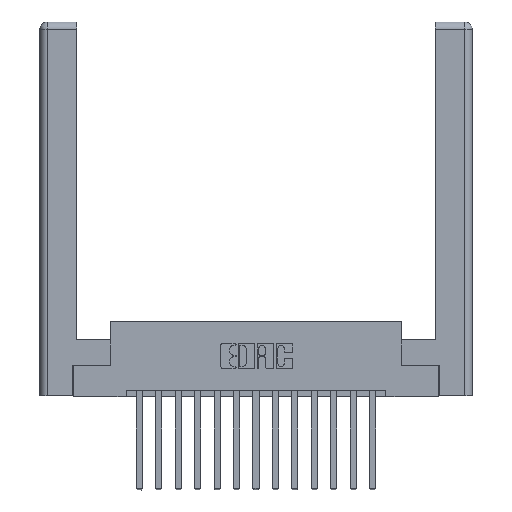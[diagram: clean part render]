
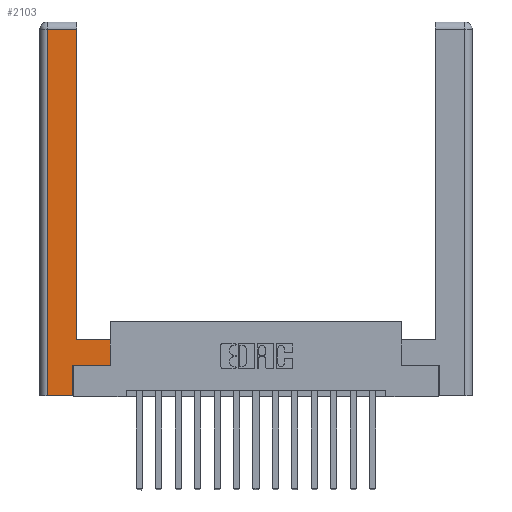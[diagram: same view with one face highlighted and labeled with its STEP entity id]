
A CAD part, top view. The second image highlights one B-rep face of the part: STEP entity #2103.
In plain terms, the highlighted planar face has unit normal (0, 0, 1).
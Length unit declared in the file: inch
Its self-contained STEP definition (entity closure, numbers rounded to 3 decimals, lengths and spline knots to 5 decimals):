
#102 = ORIENTED_EDGE ( 'NONE', *, *, #4767, .T. ) ;
#335 = ORIENTED_EDGE ( 'NONE', *, *, #12388, .T. ) ;
#626 = CARTESIAN_POINT ( 'NONE',  ( 0.295, 0.45, 0. ) ) ;
#702 = CARTESIAN_POINT ( 'NONE',  ( 0.565, 0.245, 0. ) ) ;
#772 = CARTESIAN_POINT ( 'NONE',  ( 0.0615, 0., 0. ) ) ;
#853 = LINE ( 'NONE', #11013, #13833 ) ;
#1168 = DIRECTION ( 'NONE',  ( 0., 0., -1. ) ) ;
#1185 = ORIENTED_EDGE ( 'NONE', *, *, #1315, .T. ) ;
#1315 = EDGE_CURVE ( 'NONE', #10951, #4838, #11542, .T. ) ;
#1428 = VERTEX_POINT ( 'NONE', #8576 ) ;
#2026 = CARTESIAN_POINT ( 'NONE',  ( 0.565, 0.245, 0. ) ) ;
#2069 = CARTESIAN_POINT ( 'NONE',  ( 0.565, 0.45, 0. ) ) ;
#2103 = ADVANCED_FACE ( 'NONE', ( #9346 ), #11185, .F. ) ;
#2942 = VERTEX_POINT ( 'NONE', #702 ) ;
#3181 = VERTEX_POINT ( 'NONE', #2069 ) ;
#3191 = CARTESIAN_POINT ( 'NONE',  ( 0.295, 2.94, 0. ) ) ;
#3238 = LINE ( 'NONE', #5277, #14040 ) ;
#3757 = VECTOR ( 'NONE', #6962, 39.37008 ) ;
#3889 = VECTOR ( 'NONE', #16175, 39.37008 ) ;
#4023 = DIRECTION ( 'NONE',  ( 0., -1., 0. ) ) ;
#4046 = DIRECTION ( 'NONE',  ( 0., 1., 0. ) ) ;
#4767 = EDGE_CURVE ( 'NONE', #2942, #3181, #3238, .T. ) ;
#4838 = VERTEX_POINT ( 'NONE', #772 ) ;
#5277 = CARTESIAN_POINT ( 'NONE',  ( 0.565, 0.45, 0. ) ) ;
#5651 = ORIENTED_EDGE ( 'NONE', *, *, #11709, .T. ) ;
#6051 = LINE ( 'NONE', #7286, #3889 ) ;
#6145 = DIRECTION ( 'NONE',  ( -1., 0., 0. ) ) ;
#6656 = EDGE_CURVE ( 'NONE', #7802, #1428, #9252, .T. ) ;
#6962 = DIRECTION ( 'NONE',  ( 0., 1., 0. ) ) ;
#7286 = CARTESIAN_POINT ( 'NONE',  ( 0.265, 0., 0. ) ) ;
#7357 = VECTOR ( 'NONE', #15748, 39.37008 ) ;
#7420 = CARTESIAN_POINT ( 'NONE',  ( 0., 0., 0. ) ) ;
#7625 = VECTOR ( 'NONE', #4023, 39.37008 ) ;
#7802 = VERTEX_POINT ( 'NONE', #15388 ) ;
#8325 = LINE ( 'NONE', #11782, #7357 ) ;
#8418 = AXIS2_PLACEMENT_3D ( 'NONE', #7420, #1168, #6145 ) ;
#8576 = CARTESIAN_POINT ( 'NONE',  ( 0.265, 0.245, 0. ) ) ;
#8760 = EDGE_CURVE ( 'NONE', #1428, #2942, #10164, .T. ) ;
#8949 = CARTESIAN_POINT ( 'NONE',  ( 0.0615, 0., 0. ) ) ;
#8981 = CARTESIAN_POINT ( 'NONE',  ( 0.0615, 2.94, 0. ) ) ;
#9252 = LINE ( 'NONE', #10608, #3757 ) ;
#9346 = FACE_OUTER_BOUND ( 'NONE', #14970, .T. ) ;
#9772 = VECTOR ( 'NONE', #14393, 39.37008 ) ;
#10125 = ORIENTED_EDGE ( 'NONE', *, *, #11479, .T. ) ;
#10164 = LINE ( 'NONE', #2026, #9772 ) ;
#10608 = CARTESIAN_POINT ( 'NONE',  ( 0.265, 0.245, 0. ) ) ;
#10736 = CARTESIAN_POINT ( 'NONE',  ( 0.0615, 2.94, 0. ) ) ;
#10951 = VERTEX_POINT ( 'NONE', #8981 ) ;
#11013 = CARTESIAN_POINT ( 'NONE',  ( 0.295, 3., 0. ) ) ;
#11185 = PLANE ( 'NONE',  #8418 ) ;
#11373 = VERTEX_POINT ( 'NONE', #626 ) ;
#11479 = EDGE_CURVE ( 'NONE', #11373, #15918, #853, .T. ) ;
#11542 = LINE ( 'NONE', #8949, #7625 ) ;
#11709 = EDGE_CURVE ( 'NONE', #3181, #11373, #8325, .T. ) ;
#11782 = CARTESIAN_POINT ( 'NONE',  ( 0.295, 0.45, 0. ) ) ;
#12215 = DIRECTION ( 'NONE',  ( -1., 0., 0. ) ) ;
#12388 = EDGE_CURVE ( 'NONE', #15918, #10951, #14791, .T. ) ;
#12442 = DIRECTION ( 'NONE',  ( 0., 1., 0. ) ) ;
#12627 = VECTOR ( 'NONE', #12215, 39.37008 ) ;
#12668 = ORIENTED_EDGE ( 'NONE', *, *, #6656, .T. ) ;
#13788 = ORIENTED_EDGE ( 'NONE', *, *, #15567, .T. ) ;
#13833 = VECTOR ( 'NONE', #12442, 39.37008 ) ;
#13871 = ORIENTED_EDGE ( 'NONE', *, *, #8760, .T. ) ;
#14040 = VECTOR ( 'NONE', #4046, 39.37008 ) ;
#14393 = DIRECTION ( 'NONE',  ( 1., 0., 0. ) ) ;
#14791 = LINE ( 'NONE', #10736, #12627 ) ;
#14970 = EDGE_LOOP ( 'NONE', ( #10125, #335, #1185, #13788, #12668, #13871, #102, #5651 ) ) ;
#15388 = CARTESIAN_POINT ( 'NONE',  ( 0.265, 0., 0. ) ) ;
#15567 = EDGE_CURVE ( 'NONE', #4838, #7802, #6051, .T. ) ;
#15748 = DIRECTION ( 'NONE',  ( -1., 0., 0. ) ) ;
#15918 = VERTEX_POINT ( 'NONE', #3191 ) ;
#16175 = DIRECTION ( 'NONE',  ( 1., 0., 0. ) ) ;
